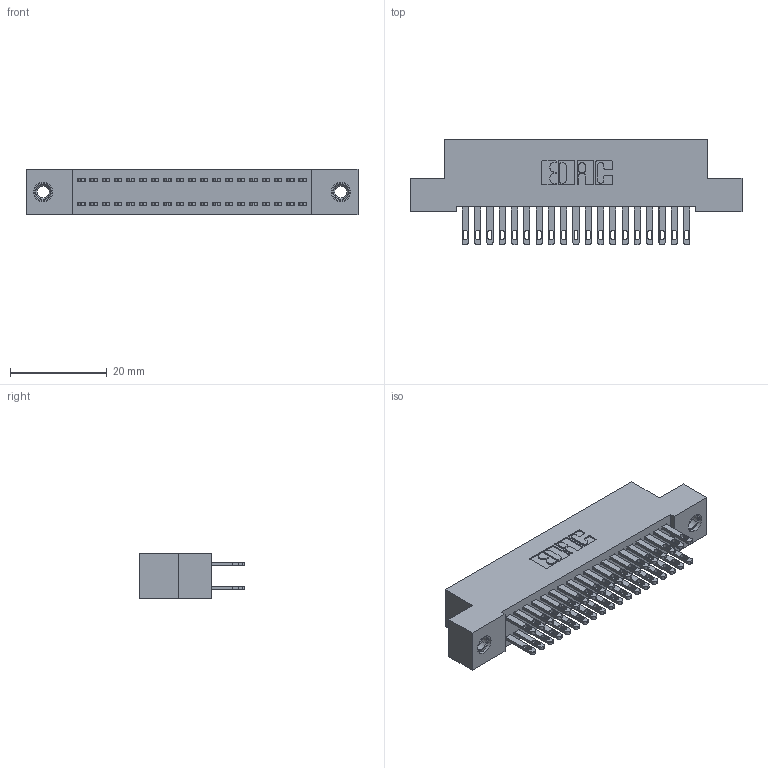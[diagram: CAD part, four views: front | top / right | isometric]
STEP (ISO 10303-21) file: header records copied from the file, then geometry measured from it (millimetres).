
FILE_DESCRIPTION (( 'STEP AP203' ), '1' );
FILE_NAME ('892-038-500-207.STEP', '2020-09-21T16:13:33', ( '' ), ( '' ), 'SwSTEP 2.0', 'SolidWorks 2020', '' );
FILE_SCHEMA (( 'CONFIG_CONTROL_DESIGN' ));
Length unit declared in the file: inch
Products named in the file (4): 345-250-001_345-250-005-103; 892-038-500-207; 842 Part_TI; 345-292-001_345-293-100
Assembly tree (41 placements, depth 2):
  892-038-500-207
    842 Part_TI
    345-292-001_345-293-100  x38
    345-250-001_345-250-005-103  x2
Bounding box: 68.58 x 21.85 x 9.4 mm (x, y, z)
Volume: 6156.5 mm3; surface area: 9844.1 mm2
Topology: 41 solids, 41 shells, 1994 faces, 6021 edges, 4006 vertices
Faces by surface type: plane 1238, cylinder 740, cone 12, torus 4
Entity records: 16182 total; most frequent: CARTESIAN_POINT 2689, ORIENTED_EDGE 2618, DIRECTION 2371, EDGE_CURVE 1309, VECTOR 1157, LINE 1157, VERTEX_POINT 868, AXIS2_PLACEMENT_3D 607
